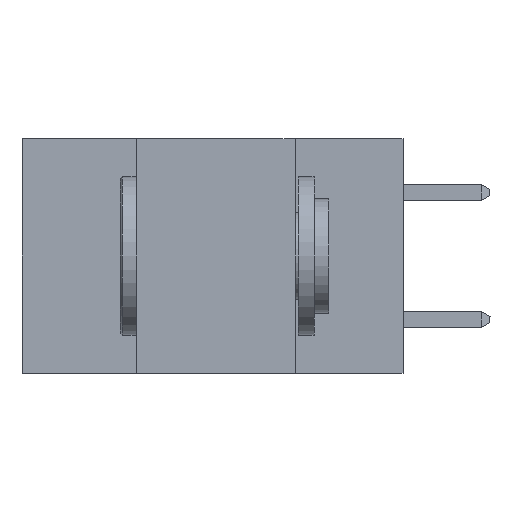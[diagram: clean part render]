
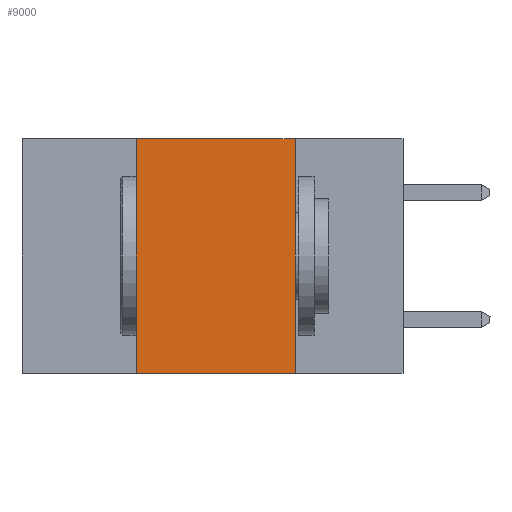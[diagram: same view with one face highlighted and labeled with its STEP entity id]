
A CAD part, left-side view. The second image highlights one B-rep face of the part: STEP entity #9000.
In plain terms, the highlighted planar face has unit normal (-1, 0, 0).
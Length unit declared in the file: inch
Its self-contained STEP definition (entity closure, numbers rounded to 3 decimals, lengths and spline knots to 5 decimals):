
#853 = DIRECTION ( 'NONE',  ( 0., -1., 0. ) ) ;
#913 = EDGE_CURVE ( 'NONE', #13043, #9216, #9476, .T. ) ;
#1297 = EDGE_CURVE ( 'NONE', #14305, #9216, #19908, .T. ) ;
#2255 = EDGE_LOOP ( 'NONE', ( #11833, #23532, #4643, #4586 ) ) ;
#2664 = EDGE_CURVE ( 'NONE', #24542, #13043, #16321, .T. ) ;
#4387 = VECTOR ( 'NONE', #23017, 39.37008 ) ;
#4586 = ORIENTED_EDGE ( 'NONE', *, *, #1297, .T. ) ;
#4643 = ORIENTED_EDGE ( 'NONE', *, *, #9748, .F. ) ;
#5722 = DIRECTION ( 'NONE',  ( 1., 0., 0. ) ) ;
#8897 = CARTESIAN_POINT ( 'NONE',  ( 0., 0.42, -0.37 ) ) ;
#9000 = ADVANCED_FACE ( 'NONE', ( #16622 ), #26844, .F. ) ;
#9216 = VERTEX_POINT ( 'NONE', #12602 ) ;
#9476 = LINE ( 'NONE', #16435, #19270 ) ;
#9748 = EDGE_CURVE ( 'NONE', #14305, #24542, #27665, .T. ) ;
#9781 = VECTOR ( 'NONE', #11137, 39.37008 ) ;
#9785 = CARTESIAN_POINT ( 'NONE',  ( 0., 0.6, 0. ) ) ;
#9962 = CARTESIAN_POINT ( 'NONE',  ( 0., 0.6, -0.37 ) ) ;
#10339 = AXIS2_PLACEMENT_3D ( 'NONE', #9785, #5722, #18795 ) ;
#11137 = DIRECTION ( 'NONE',  ( 0., 0., 1. ) ) ;
#11769 = CARTESIAN_POINT ( 'NONE',  ( 0., 0.17, 0. ) ) ;
#11833 = ORIENTED_EDGE ( 'NONE', *, *, #913, .F. ) ;
#12602 = CARTESIAN_POINT ( 'NONE',  ( 0., 0.17, -0.37 ) ) ;
#13043 = VERTEX_POINT ( 'NONE', #11769 ) ;
#13225 = CARTESIAN_POINT ( 'NONE',  ( 0., 0.42, 0. ) ) ;
#14305 = VERTEX_POINT ( 'NONE', #8897 ) ;
#14434 = DIRECTION ( 'NONE',  ( 0., 0., -1. ) ) ;
#16321 = LINE ( 'NONE', #17600, #24069 ) ;
#16435 = CARTESIAN_POINT ( 'NONE',  ( 0., 0.17, 0. ) ) ;
#16622 = FACE_OUTER_BOUND ( 'NONE', #2255, .T. ) ;
#17600 = CARTESIAN_POINT ( 'NONE',  ( 0., 0.6, 0. ) ) ;
#18795 = DIRECTION ( 'NONE',  ( 0., 0., -1. ) ) ;
#19270 = VECTOR ( 'NONE', #14434, 39.37008 ) ;
#19908 = LINE ( 'NONE', #9962, #4387 ) ;
#23017 = DIRECTION ( 'NONE',  ( 0., -1., 0. ) ) ;
#23532 = ORIENTED_EDGE ( 'NONE', *, *, #2664, .F. ) ;
#24069 = VECTOR ( 'NONE', #853, 39.37008 ) ;
#24542 = VERTEX_POINT ( 'NONE', #25473 ) ;
#25473 = CARTESIAN_POINT ( 'NONE',  ( 0., 0.42, 0. ) ) ;
#26844 = PLANE ( 'NONE',  #10339 ) ;
#27665 = LINE ( 'NONE', #13225, #9781 ) ;
